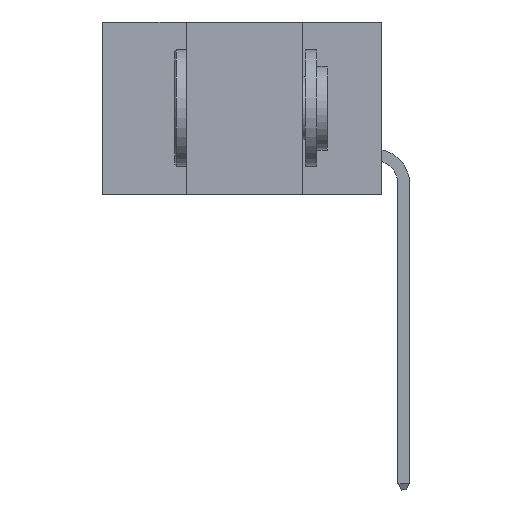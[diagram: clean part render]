
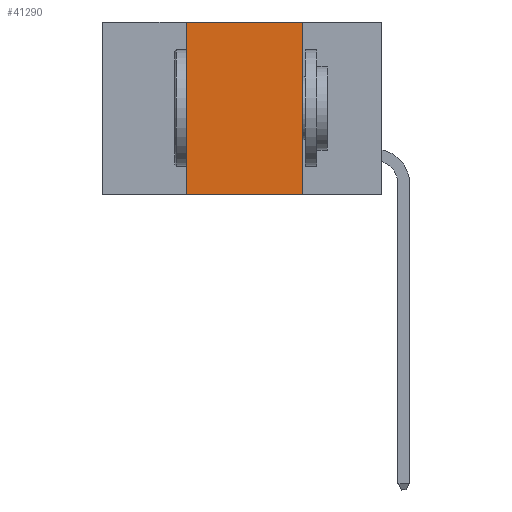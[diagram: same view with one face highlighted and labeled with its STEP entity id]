
A CAD part, left-side view. The second image highlights one B-rep face of the part: STEP entity #41290.
In plain terms, the highlighted planar face has unit normal (-1, 0, 0).
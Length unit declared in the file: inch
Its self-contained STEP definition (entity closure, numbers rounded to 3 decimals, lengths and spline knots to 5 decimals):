
#149 = ORIENTED_EDGE ( 'NONE', *, *, #9445, .F. ) ;
#917 = VECTOR ( 'NONE', #49070, 39.37008 ) ;
#1362 = VECTOR ( 'NONE', #14376, 39.37008 ) ;
#1395 = VECTOR ( 'NONE', #1841, 39.37008 ) ;
#1841 = DIRECTION ( 'NONE',  ( 0., -1., 0. ) ) ;
#2007 = AXIS2_PLACEMENT_3D ( 'NONE', #3263, #44394, #22018 ) ;
#3263 = CARTESIAN_POINT ( 'NONE',  ( 0., 0.6, 0. ) ) ;
#3887 = VERTEX_POINT ( 'NONE', #49010 ) ;
#4118 = EDGE_CURVE ( 'NONE', #19895, #29013, #44243, .T. ) ;
#5681 = CARTESIAN_POINT ( 'NONE',  ( 0., 0.6, 0. ) ) ;
#7042 = CARTESIAN_POINT ( 'NONE',  ( 0., 0.42, 0. ) ) ;
#9445 = EDGE_CURVE ( 'NONE', #34879, #3887, #36537, .T. ) ;
#9941 = ORIENTED_EDGE ( 'NONE', *, *, #31686, .F. ) ;
#10724 = EDGE_LOOP ( 'NONE', ( #15386, #149, #9941, #17929 ) ) ;
#11111 = VECTOR ( 'NONE', #39693, 39.37008 ) ;
#14273 = PLANE ( 'NONE',  #2007 ) ;
#14376 = DIRECTION ( 'NONE',  ( 0., -1., 0. ) ) ;
#15386 = ORIENTED_EDGE ( 'NONE', *, *, #43873, .F. ) ;
#17929 = ORIENTED_EDGE ( 'NONE', *, *, #4118, .T. ) ;
#19895 = VERTEX_POINT ( 'NONE', #47465 ) ;
#22018 = DIRECTION ( 'NONE',  ( 0., 0., -1. ) ) ;
#26281 = CARTESIAN_POINT ( 'NONE',  ( 0., 0.6, -0.37 ) ) ;
#29013 = VERTEX_POINT ( 'NONE', #31092 ) ;
#29398 = CARTESIAN_POINT ( 'NONE',  ( 0., 0.42, 0. ) ) ;
#31092 = CARTESIAN_POINT ( 'NONE',  ( 0., 0.17, -0.37 ) ) ;
#31686 = EDGE_CURVE ( 'NONE', #19895, #34879, #34829, .T. ) ;
#33975 = FACE_OUTER_BOUND ( 'NONE', #10724, .T. ) ;
#34829 = LINE ( 'NONE', #7042, #917 ) ;
#34879 = VERTEX_POINT ( 'NONE', #29398 ) ;
#36537 = LINE ( 'NONE', #5681, #1395 ) ;
#37224 = LINE ( 'NONE', #46636, #11111 ) ;
#39693 = DIRECTION ( 'NONE',  ( 0., 0., -1. ) ) ;
#41290 = ADVANCED_FACE ( 'NONE', ( #33975 ), #14273, .F. ) ;
#43873 = EDGE_CURVE ( 'NONE', #3887, #29013, #37224, .T. ) ;
#44243 = LINE ( 'NONE', #26281, #1362 ) ;
#44394 = DIRECTION ( 'NONE',  ( 1., 0., 0. ) ) ;
#46636 = CARTESIAN_POINT ( 'NONE',  ( 0., 0.17, 0. ) ) ;
#47465 = CARTESIAN_POINT ( 'NONE',  ( 0., 0.42, -0.37 ) ) ;
#49010 = CARTESIAN_POINT ( 'NONE',  ( 0., 0.17, 0. ) ) ;
#49070 = DIRECTION ( 'NONE',  ( 0., 0., 1. ) ) ;
